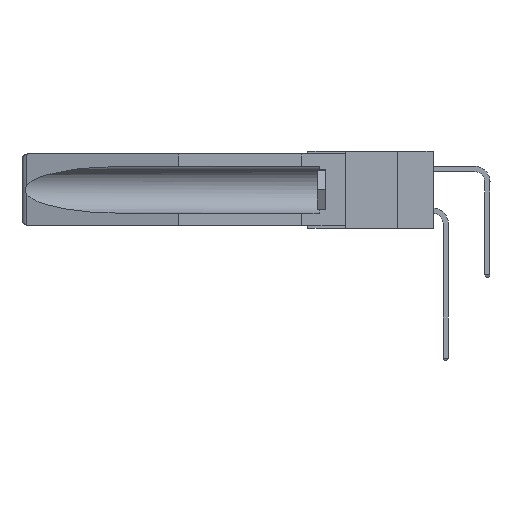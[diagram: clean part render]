
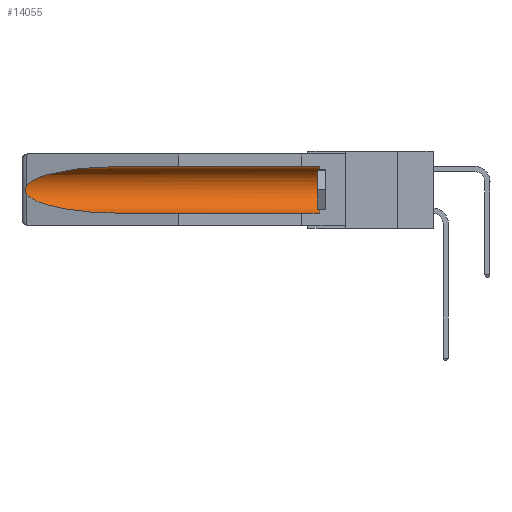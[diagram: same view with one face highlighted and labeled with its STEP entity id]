
A CAD part, left-side view. The second image highlights one B-rep face of the part: STEP entity #14055.
In plain terms, the highlighted cylindrical face has radius 2.857 mm (diameter 5.715 mm), a partial arc.
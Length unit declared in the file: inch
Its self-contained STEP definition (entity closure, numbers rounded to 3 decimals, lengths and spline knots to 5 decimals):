
#636 = CARTESIAN_POINT ( 'NONE',  ( 0.155, 1.07973, -0.284 ) ) ;
#1093 = CARTESIAN_POINT ( 'NONE',  ( 0.155, 1.07973, -0.059 ) ) ;
#1201 = LINE ( 'NONE', #1860, #8113 ) ;
#1532 = CARTESIAN_POINT ( 'NONE',  ( 0.26537, 1.52718, -0.19328 ) ) ;
#1838 = VERTEX_POINT ( 'NONE', #14390 ) ;
#1860 = CARTESIAN_POINT ( 'NONE',  ( 0.155, -0.30754, -0.059 ) ) ;
#1971 = EDGE_CURVE ( 'NONE', #1838, #13150, #5900, .T. ) ;
#2042 = DIRECTION ( 'NONE',  ( 0., 1., 0. ) ) ;
#2060 = EDGE_CURVE ( 'NONE', #15720, #17221, #5491, .T. ) ;
#2156 = CARTESIAN_POINT ( 'NONE',  ( 0.26654, 1.53092, -0.15636 ) ) ;
#2330 = CARTESIAN_POINT ( 'NONE',  ( 0.155, -0.30754, -0.284 ) ) ;
#2360 = EDGE_LOOP ( 'NONE', ( #13737, #13432, #2724, #7026, #17930, #15137 ) ) ;
#2724 = ORIENTED_EDGE ( 'NONE', *, *, #14374, .T. ) ;
#2763 = B_SPLINE_CURVE_WITH_KNOTS ( 'NONE', 3,
 ( #4880, #7813, #2156, #3565, #7685, #10672, #4816, #14635, #13483, #5070 ),
 .UNSPECIFIED., .F., .F.,
 ( 4, 2, 2, 2, 4 ),
 ( 0., 0.00029, 0.00058, 0.00087, 0.00117 ),
 .UNSPECIFIED. ) ;
#3195 = VERTEX_POINT ( 'NONE', #4809 ) ;
#3319 =( BOUNDED_CURVE ( )  B_SPLINE_CURVE ( 3, ( #1532, #10026, #16262, #636 ),
 .UNSPECIFIED., .F., .F. ) 
 B_SPLINE_CURVE_WITH_KNOTS ( ( 4, 4 ),
 ( 0.1948, 1.5708 ),
 .UNSPECIFIED. ) 
 CURVE ( )  GEOMETRIC_REPRESENTATION_ITEM ( )  RATIONAL_B_SPLINE_CURVE ( ( 1., 0.848, 0.848, 1. ) ) 
 REPRESENTATION_ITEM ( '' )  );
#3565 = CARTESIAN_POINT ( 'NONE',  ( 0.2673, 1.5327, -0.16383 ) ) ;
#4155 = CARTESIAN_POINT ( 'NONE',  ( 0.155, 1.07973, -0.059 ) ) ;
#4461 = DIRECTION ( 'NONE',  ( 0., 1., 0. ) ) ;
#4809 = CARTESIAN_POINT ( 'NONE',  ( 0.155, 0.126, -0.059 ) ) ;
#4816 = CARTESIAN_POINT ( 'NONE',  ( 0.2673, 1.53269, -0.17917 ) ) ;
#4880 = CARTESIAN_POINT ( 'NONE',  ( 0.26537, 1.52718, -0.14972 ) ) ;
#5070 = CARTESIAN_POINT ( 'NONE',  ( 0.26537, 1.52718, -0.19328 ) ) ;
#5391 = VERTEX_POINT ( 'NONE', #12402 ) ;
#5491 =( BOUNDED_CURVE ( )  B_SPLINE_CURVE ( 3, ( #4155, #7162, #15300, #18144 ),
 .UNSPECIFIED., .F., .F. ) 
 B_SPLINE_CURVE_WITH_KNOTS ( ( 4, 4 ),
 ( 4.71239, 6.08839 ),
 .UNSPECIFIED. ) 
 CURVE ( )  GEOMETRIC_REPRESENTATION_ITEM ( )  RATIONAL_B_SPLINE_CURVE ( ( 1., 0.848, 0.848, 1. ) ) 
 REPRESENTATION_ITEM ( '' )  );
#5900 = LINE ( 'NONE', #2330, #8123 ) ;
#7008 = EDGE_CURVE ( 'NONE', #1838, #3195, #11511, .T. ) ;
#7024 = CARTESIAN_POINT ( 'NONE',  ( 0.26537, 1.52718, -0.14972 ) ) ;
#7026 = ORIENTED_EDGE ( 'NONE', *, *, #1971, .F. ) ;
#7162 = CARTESIAN_POINT ( 'NONE',  ( 0.21114, 1.30732, -0.059 ) ) ;
#7685 = CARTESIAN_POINT ( 'NONE',  ( 0.2675, 1.53308, -0.16763 ) ) ;
#7813 = CARTESIAN_POINT ( 'NONE',  ( 0.26597, 1.52961, -0.15275 ) ) ;
#8113 = VECTOR ( 'NONE', #2042, 39.37008 ) ;
#8123 = VECTOR ( 'NONE', #14996, 39.37008 ) ;
#8537 = CARTESIAN_POINT ( 'NONE',  ( 0.155, 1.07973, -0.284 ) ) ;
#10026 = CARTESIAN_POINT ( 'NONE',  ( 0.25451, 1.48313, -0.24835 ) ) ;
#10672 = CARTESIAN_POINT ( 'NONE',  ( 0.2675, 1.53308, -0.17534 ) ) ;
#10870 = DIRECTION ( 'NONE',  ( 0., -1., 0. ) ) ;
#10961 = EDGE_CURVE ( 'NONE', #3195, #15720, #1201, .T. ) ;
#11506 = CYLINDRICAL_SURFACE ( 'NONE', #15684, 0.1125 ) ;
#11511 = CIRCLE ( 'NONE', #17459, 0.1125 ) ;
#12402 = CARTESIAN_POINT ( 'NONE',  ( 0.26537, 1.52718, -0.19328 ) ) ;
#13150 = VERTEX_POINT ( 'NONE', #8537 ) ;
#13432 = ORIENTED_EDGE ( 'NONE', *, *, #13790, .T. ) ;
#13483 = CARTESIAN_POINT ( 'NONE',  ( 0.26597, 1.5296, -0.19026 ) ) ;
#13737 = ORIENTED_EDGE ( 'NONE', *, *, #2060, .T. ) ;
#13790 = EDGE_CURVE ( 'NONE', #17221, #5391, #2763, .T. ) ;
#14055 = ADVANCED_FACE ( 'NONE', ( #15415 ), #11506, .F. ) ;
#14374 = EDGE_CURVE ( 'NONE', #5391, #13150, #3319, .T. ) ;
#14390 = CARTESIAN_POINT ( 'NONE',  ( 0.155, 0.126, -0.284 ) ) ;
#14635 = CARTESIAN_POINT ( 'NONE',  ( 0.26655, 1.53094, -0.18657 ) ) ;
#14779 = DIRECTION ( 'NONE',  ( 0., 0., 1. ) ) ;
#14996 = DIRECTION ( 'NONE',  ( 0., 1., 0. ) ) ;
#15137 = ORIENTED_EDGE ( 'NONE', *, *, #10961, .T. ) ;
#15300 = CARTESIAN_POINT ( 'NONE',  ( 0.25451, 1.48313, -0.09465 ) ) ;
#15415 = FACE_OUTER_BOUND ( 'NONE', #2360, .T. ) ;
#15643 = CARTESIAN_POINT ( 'NONE',  ( 0.155, -0.30754, -0.1715 ) ) ;
#15684 = AXIS2_PLACEMENT_3D ( 'NONE', #15643, #4461, #17102 ) ;
#15720 = VERTEX_POINT ( 'NONE', #1093 ) ;
#16262 = CARTESIAN_POINT ( 'NONE',  ( 0.21114, 1.30732, -0.284 ) ) ;
#16306 = CARTESIAN_POINT ( 'NONE',  ( 0.155, 0.126, -0.1715 ) ) ;
#17102 = DIRECTION ( 'NONE',  ( 0., 0., 1. ) ) ;
#17221 = VERTEX_POINT ( 'NONE', #7024 ) ;
#17459 = AXIS2_PLACEMENT_3D ( 'NONE', #16306, #10870, #14779 ) ;
#17930 = ORIENTED_EDGE ( 'NONE', *, *, #7008, .T. ) ;
#18144 = CARTESIAN_POINT ( 'NONE',  ( 0.26537, 1.52718, -0.14972 ) ) ;
